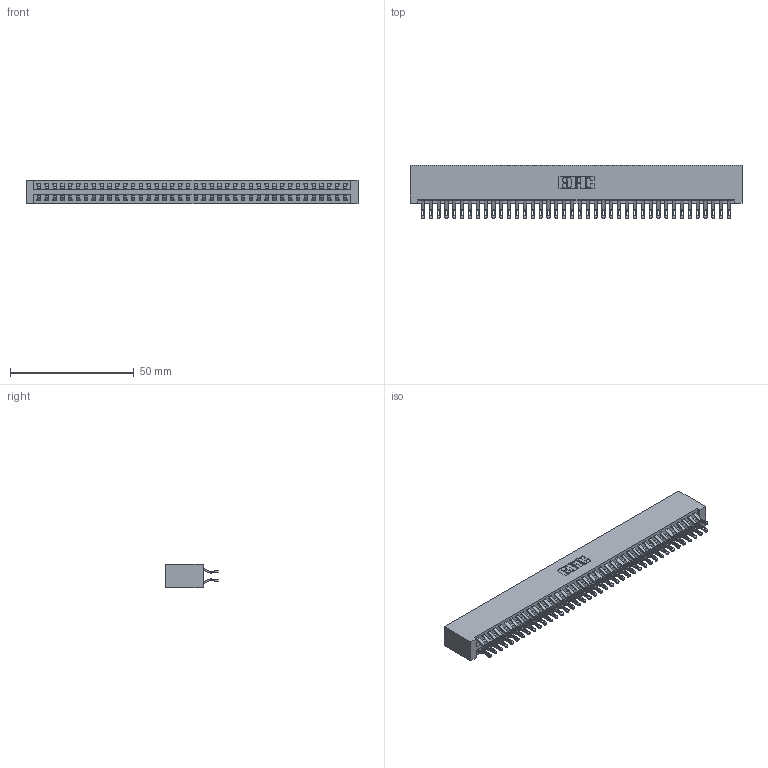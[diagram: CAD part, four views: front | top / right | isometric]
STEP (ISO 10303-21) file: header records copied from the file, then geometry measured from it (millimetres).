
FILE_DESCRIPTION (( 'STEP AP203' ), '1' );
FILE_NAME ('396-080-555-201.STEP', '2018-09-09T21:09:25', ( '' ), ( '' ), 'SwSTEP 2.0', 'SolidWorks 2016', '' );
FILE_SCHEMA (( 'CONFIG_CONTROL_DESIGN' ));
Length unit declared in the file: inch
Products named in the file (3): 346 Part_No Mounting Lugs; 345-292-001_555 Tail; 396-080-555-201
Assembly tree (81 placements, depth 2):
  396-080-555-201
    346 Part_No Mounting Lugs
    345-292-001_555 Tail  x80
Bounding box: 134.24 x 21.46 x 9.4 mm (x, y, z)
Volume: 13879.8 mm3; surface area: 20037.6 mm2
Topology: 81 solids, 81 shells, 4754 faces, 14945 edges, 9962 vertices
Faces by surface type: plane 2712, cylinder 2042
Entity records: 26423 total; most frequent: CARTESIAN_POINT 4390, ORIENTED_EDGE 4294, DIRECTION 3883, EDGE_CURVE 2147, VECTOR 1843, LINE 1843, VERTEX_POINT 1430, AXIS2_PLACEMENT_3D 1020
